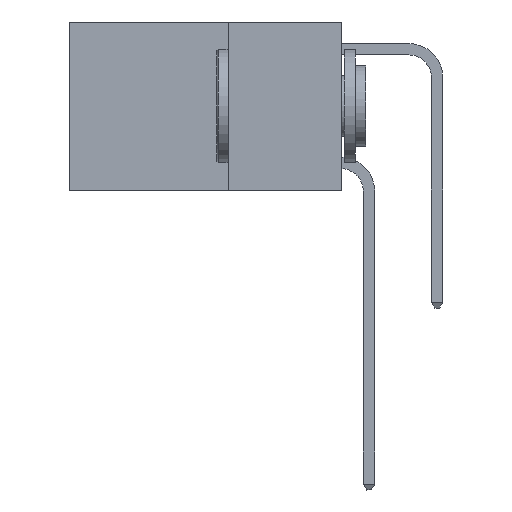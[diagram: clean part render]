
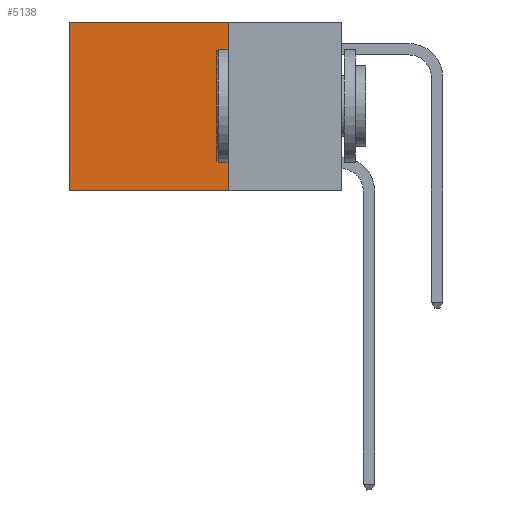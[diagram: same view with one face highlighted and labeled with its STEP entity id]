
A CAD part, left-side view. The second image highlights one B-rep face of the part: STEP entity #5138.
In plain terms, the highlighted planar face has unit normal (-1, 0, 0).
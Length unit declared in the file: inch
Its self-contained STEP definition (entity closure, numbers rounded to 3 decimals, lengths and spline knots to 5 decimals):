
#22 = VECTOR ( 'NONE', #2908, 39.37008 ) ;
#573 = CARTESIAN_POINT ( 'NONE',  ( 0.2625, 0.25, 0. ) ) ;
#1015 = VERTEX_POINT ( 'NONE', #11758 ) ;
#1478 = CARTESIAN_POINT ( 'NONE',  ( 0.2625, 0.25, 0. ) ) ;
#1790 = EDGE_LOOP ( 'NONE', ( #16130, #17874, #15873, #3991 ) ) ;
#2908 = DIRECTION ( 'NONE',  ( 0., 1., 0. ) ) ;
#3261 = CARTESIAN_POINT ( 'NONE',  ( 0.2625, 0.25, -0.37 ) ) ;
#3978 = VERTEX_POINT ( 'NONE', #3261 ) ;
#3991 = ORIENTED_EDGE ( 'NONE', *, *, #4660, .T. ) ;
#4660 = EDGE_CURVE ( 'NONE', #12122, #1015, #14504, .T. ) ;
#4930 = DIRECTION ( 'NONE',  ( 0., 0., -1. ) ) ;
#5138 = ADVANCED_FACE ( 'NONE', ( #5470 ), #8664, .F. ) ;
#5470 = FACE_OUTER_BOUND ( 'NONE', #1790, .T. ) ;
#5600 = VECTOR ( 'NONE', #10560, 39.37008 ) ;
#6231 = LINE ( 'NONE', #573, #5600 ) ;
#6583 = CARTESIAN_POINT ( 'NONE',  ( 0.2625, 0.6, 0. ) ) ;
#7404 = EDGE_CURVE ( 'NONE', #1015, #16140, #16731, .T. ) ;
#8664 = PLANE ( 'NONE',  #16835 ) ;
#10017 = EDGE_CURVE ( 'NONE', #12122, #3978, #6231, .T. ) ;
#10560 = DIRECTION ( 'NONE',  ( 0., 0., -1. ) ) ;
#10692 = CARTESIAN_POINT ( 'NONE',  ( 0.2625, 0.25, 0. ) ) ;
#11427 = DIRECTION ( 'NONE',  ( 0., 0., -1. ) ) ;
#11758 = CARTESIAN_POINT ( 'NONE',  ( 0.2625, 0.6, 0. ) ) ;
#11910 = LINE ( 'NONE', #17822, #13379 ) ;
#12122 = VERTEX_POINT ( 'NONE', #10692 ) ;
#12271 = CARTESIAN_POINT ( 'NONE',  ( 0.2625, 0.6, -0.37 ) ) ;
#13327 = DIRECTION ( 'NONE',  ( 0., 1., 0. ) ) ;
#13379 = VECTOR ( 'NONE', #13327, 39.37008 ) ;
#14185 = CARTESIAN_POINT ( 'NONE',  ( 0.2625, 0.25, 0. ) ) ;
#14504 = LINE ( 'NONE', #1478, #22 ) ;
#15729 = DIRECTION ( 'NONE',  ( 1., 0., 0. ) ) ;
#15873 = ORIENTED_EDGE ( 'NONE', *, *, #10017, .F. ) ;
#15929 = EDGE_CURVE ( 'NONE', #3978, #16140, #11910, .T. ) ;
#16130 = ORIENTED_EDGE ( 'NONE', *, *, #7404, .T. ) ;
#16140 = VERTEX_POINT ( 'NONE', #12271 ) ;
#16281 = VECTOR ( 'NONE', #4930, 39.37008 ) ;
#16731 = LINE ( 'NONE', #6583, #16281 ) ;
#16835 = AXIS2_PLACEMENT_3D ( 'NONE', #14185, #15729, #11427 ) ;
#17822 = CARTESIAN_POINT ( 'NONE',  ( 0.2625, 0.25, -0.37 ) ) ;
#17874 = ORIENTED_EDGE ( 'NONE', *, *, #15929, .F. ) ;
